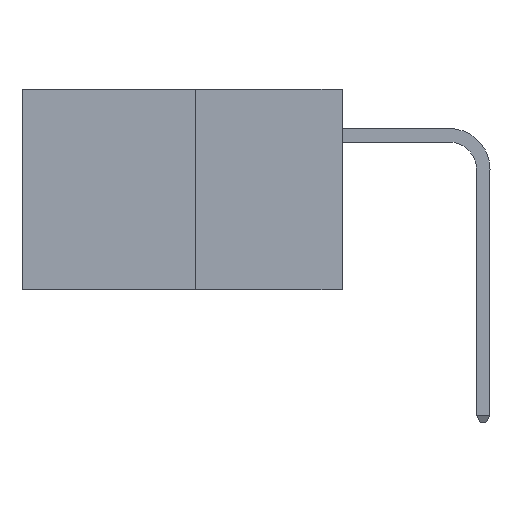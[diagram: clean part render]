
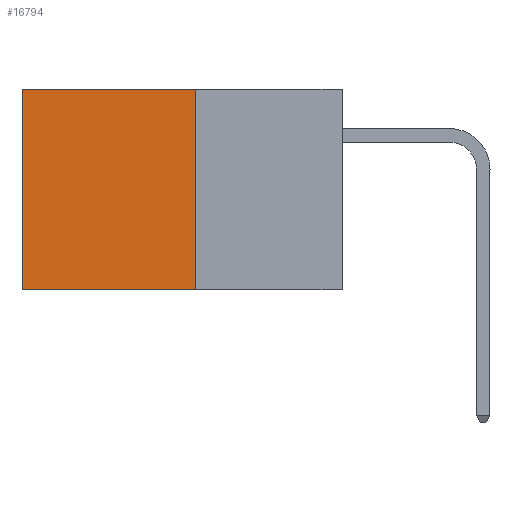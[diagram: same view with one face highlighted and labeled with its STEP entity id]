
A CAD part, left-side view. The second image highlights one B-rep face of the part: STEP entity #16794.
In plain terms, the highlighted planar face has unit normal (-1, 0, 0).
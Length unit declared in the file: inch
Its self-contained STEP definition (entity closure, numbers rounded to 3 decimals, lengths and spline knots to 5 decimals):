
#112 = CARTESIAN_POINT ( 'NONE',  ( 0.277, 0.27, -0.37 ) ) ;
#246 = LINE ( 'NONE', #8263, #7203 ) ;
#1366 = DIRECTION ( 'NONE',  ( 0., 1., 0. ) ) ;
#2466 = ORIENTED_EDGE ( 'NONE', *, *, #14243, .F. ) ;
#2791 = EDGE_LOOP ( 'NONE', ( #5075, #2466, #7829, #4892 ) ) ;
#3429 = VECTOR ( 'NONE', #8243, 39.37008 ) ;
#3688 = DIRECTION ( 'NONE',  ( 0., 0., -1. ) ) ;
#4297 = DIRECTION ( 'NONE',  ( 1., 0., 0. ) ) ;
#4892 = ORIENTED_EDGE ( 'NONE', *, *, #13562, .T. ) ;
#5075 = ORIENTED_EDGE ( 'NONE', *, *, #13351, .T. ) ;
#5182 = VERTEX_POINT ( 'NONE', #11898 ) ;
#7037 = VERTEX_POINT ( 'NONE', #14192 ) ;
#7203 = VECTOR ( 'NONE', #1366, 39.37008 ) ;
#7829 = ORIENTED_EDGE ( 'NONE', *, *, #9860, .F. ) ;
#8051 = CARTESIAN_POINT ( 'NONE',  ( 0.277, 0.59, -0.37 ) ) ;
#8211 = VERTEX_POINT ( 'NONE', #15252 ) ;
#8243 = DIRECTION ( 'NONE',  ( 0., 1., 0. ) ) ;
#8263 = CARTESIAN_POINT ( 'NONE',  ( 0.277, 0.27, 0. ) ) ;
#9206 = VERTEX_POINT ( 'NONE', #8051 ) ;
#9392 = DIRECTION ( 'NONE',  ( 0., 0., -1. ) ) ;
#9848 = PLANE ( 'NONE',  #11439 ) ;
#9860 = EDGE_CURVE ( 'NONE', #8211, #7037, #15607, .T. ) ;
#10709 = VECTOR ( 'NONE', #3688, 39.37008 ) ;
#10821 = LINE ( 'NONE', #15222, #3429 ) ;
#11150 = FACE_OUTER_BOUND ( 'NONE', #2791, .T. ) ;
#11439 = AXIS2_PLACEMENT_3D ( 'NONE', #112, #4297, #14064 ) ;
#11898 = CARTESIAN_POINT ( 'NONE',  ( 0.277, 0.59, 0. ) ) ;
#11921 = VECTOR ( 'NONE', #9392, 39.37008 ) ;
#13351 = EDGE_CURVE ( 'NONE', #5182, #9206, #14428, .T. ) ;
#13562 = EDGE_CURVE ( 'NONE', #8211, #5182, #246, .T. ) ;
#14064 = DIRECTION ( 'NONE',  ( 0., 0., -1. ) ) ;
#14192 = CARTESIAN_POINT ( 'NONE',  ( 0.277, 0.27, -0.37 ) ) ;
#14243 = EDGE_CURVE ( 'NONE', #7037, #9206, #10821, .T. ) ;
#14428 = LINE ( 'NONE', #17565, #10709 ) ;
#15222 = CARTESIAN_POINT ( 'NONE',  ( 0.277, 0.27, -0.37 ) ) ;
#15252 = CARTESIAN_POINT ( 'NONE',  ( 0.277, 0.27, 0. ) ) ;
#15607 = LINE ( 'NONE', #16340, #11921 ) ;
#16340 = CARTESIAN_POINT ( 'NONE',  ( 0.277, 0.27, -0.37 ) ) ;
#16794 = ADVANCED_FACE ( 'NONE', ( #11150 ), #9848, .F. ) ;
#17565 = CARTESIAN_POINT ( 'NONE',  ( 0.277, 0.59, -0.37 ) ) ;
